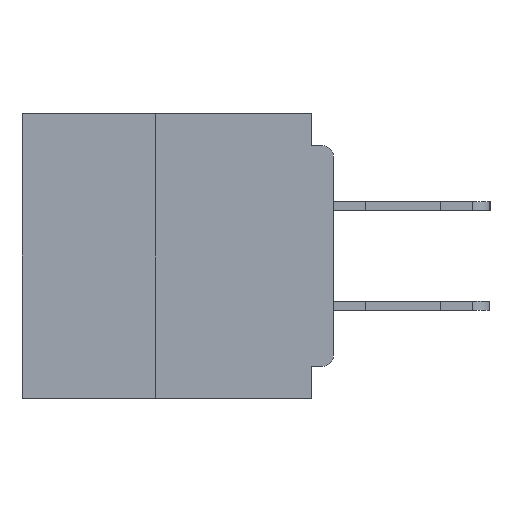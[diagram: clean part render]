
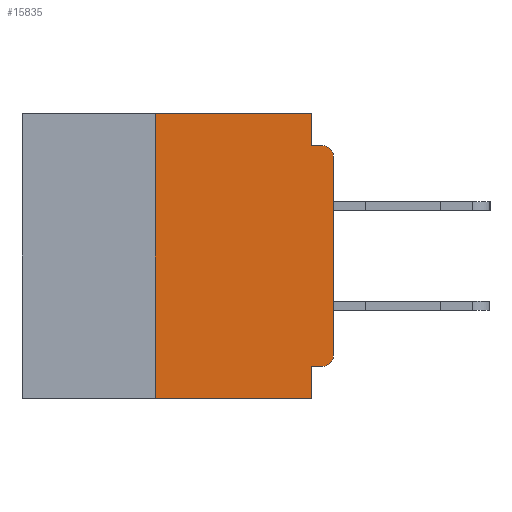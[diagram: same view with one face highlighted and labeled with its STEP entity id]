
A CAD part, left-side view. The second image highlights one B-rep face of the part: STEP entity #15835.
In plain terms, the highlighted planar face has unit normal (-1, 0, 0).
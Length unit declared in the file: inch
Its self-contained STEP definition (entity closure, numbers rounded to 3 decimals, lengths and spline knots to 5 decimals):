
#184 = VERTEX_POINT ( 'NONE', #32863 ) ;
#458 = CARTESIAN_POINT ( 'NONE',  ( 0., 0.015, -0.045 ) ) ;
#2667 = CARTESIAN_POINT ( 'NONE',  ( 0., 0.031, 0. ) ) ;
#2810 = FACE_OUTER_BOUND ( 'NONE', #41546, .T. ) ;
#3434 = CIRCLE ( 'NONE', #31598, 0.015 ) ;
#3658 = VERTEX_POINT ( 'NONE', #49305 ) ;
#4244 = CARTESIAN_POINT ( 'NONE',  ( 0., 0.437, 0. ) ) ;
#4909 = CARTESIAN_POINT ( 'NONE',  ( 0., 0.25, -0.4 ) ) ;
#6077 = ORIENTED_EDGE ( 'NONE', *, *, #34252, .F. ) ;
#7349 = LINE ( 'NONE', #2667, #27005 ) ;
#7924 = ORIENTED_EDGE ( 'NONE', *, *, #21182, .T. ) ;
#8232 = PLANE ( 'NONE',  #28793 ) ;
#9226 = EDGE_CURVE ( 'NONE', #35657, #3658, #7349, .T. ) ;
#10929 = VERTEX_POINT ( 'NONE', #26954 ) ;
#10947 = DIRECTION ( 'NONE',  ( 0., 0., 1. ) ) ;
#11020 = CARTESIAN_POINT ( 'NONE',  ( 0., 0., -0.34 ) ) ;
#11292 = EDGE_CURVE ( 'NONE', #10929, #184, #44527, .T. ) ;
#11544 = LINE ( 'NONE', #22974, #29898 ) ;
#11643 = ORIENTED_EDGE ( 'NONE', *, *, #29785, .F. ) ;
#12203 = DIRECTION ( 'NONE',  ( 0., 0., -1. ) ) ;
#12277 = ORIENTED_EDGE ( 'NONE', *, *, #48271, .F. ) ;
#13813 = LINE ( 'NONE', #38050, #43877 ) ;
#14488 = VECTOR ( 'NONE', #44711, 39.37008 ) ;
#15175 = DIRECTION ( 'NONE',  ( 0., -1., 0. ) ) ;
#15835 = ADVANCED_FACE ( 'NONE', ( #2810 ), #8232, .F. ) ;
#17308 = VECTOR ( 'NONE', #38250, 39.37008 ) ;
#17671 = CARTESIAN_POINT ( 'NONE',  ( 0., 0., -0.045 ) ) ;
#18034 = CARTESIAN_POINT ( 'NONE',  ( 0., 0.015, -0.06 ) ) ;
#19011 = VECTOR ( 'NONE', #10947, 39.37008 ) ;
#19071 = ORIENTED_EDGE ( 'NONE', *, *, #39873, .F. ) ;
#21097 = CARTESIAN_POINT ( 'NONE',  ( 0., 0.015, -0.34 ) ) ;
#21182 = EDGE_CURVE ( 'NONE', #34264, #40122, #50197, .T. ) ;
#21324 = CARTESIAN_POINT ( 'NONE',  ( 0., 0., -0.355 ) ) ;
#21983 = DIRECTION ( 'NONE',  ( 0., 0., -1. ) ) ;
#22974 = CARTESIAN_POINT ( 'NONE',  ( 0., 0.437, -0.4 ) ) ;
#23741 = LINE ( 'NONE', #4909, #42085 ) ;
#23980 = ORIENTED_EDGE ( 'NONE', *, *, #47363, .T. ) ;
#24059 = AXIS2_PLACEMENT_3D ( 'NONE', #18034, #45352, #21983 ) ;
#24980 = DIRECTION ( 'NONE',  ( 0., 0., -1. ) ) ;
#26954 = CARTESIAN_POINT ( 'NONE',  ( 0., 0.015, -0.355 ) ) ;
#27005 = VECTOR ( 'NONE', #34107, 39.37008 ) ;
#27513 = CIRCLE ( 'NONE', #24059, 0.015 ) ;
#28793 = AXIS2_PLACEMENT_3D ( 'NONE', #4244, #35649, #12203 ) ;
#29660 = VECTOR ( 'NONE', #45003, 39.37008 ) ;
#29785 = EDGE_CURVE ( 'NONE', #3658, #34527, #40076, .T. ) ;
#29898 = VECTOR ( 'NONE', #15175, 39.37008 ) ;
#30170 = CARTESIAN_POINT ( 'NONE',  ( 0., 0.25, 0. ) ) ;
#30468 = CARTESIAN_POINT ( 'NONE',  ( 0., 0., 0. ) ) ;
#31248 = ORIENTED_EDGE ( 'NONE', *, *, #46594, .T. ) ;
#31598 = AXIS2_PLACEMENT_3D ( 'NONE', #21097, #48409, #24980 ) ;
#32863 = CARTESIAN_POINT ( 'NONE',  ( 0., 0.031, -0.355 ) ) ;
#33064 = CARTESIAN_POINT ( 'NONE',  ( 0., 0.031, -0.4 ) ) ;
#34107 = DIRECTION ( 'NONE',  ( 0., 0., -1. ) ) ;
#34252 = EDGE_CURVE ( 'NONE', #48262, #35657, #48514, .T. ) ;
#34264 = VERTEX_POINT ( 'NONE', #11020 ) ;
#34327 = CARTESIAN_POINT ( 'NONE',  ( 0., 0.437, 0. ) ) ;
#34527 = VERTEX_POINT ( 'NONE', #458 ) ;
#34931 = ORIENTED_EDGE ( 'NONE', *, *, #9226, .F. ) ;
#35649 = DIRECTION ( 'NONE',  ( 1., 0., 0. ) ) ;
#35657 = VERTEX_POINT ( 'NONE', #45687 ) ;
#36324 = EDGE_CURVE ( 'NONE', #39149, #37345, #11544, .T. ) ;
#37345 = VERTEX_POINT ( 'NONE', #33064 ) ;
#37460 = CARTESIAN_POINT ( 'NONE',  ( 0., 0., -0.06 ) ) ;
#38050 = CARTESIAN_POINT ( 'NONE',  ( 0., 0.031, -0.4 ) ) ;
#38250 = DIRECTION ( 'NONE',  ( 0., -1., 0. ) ) ;
#39149 = VERTEX_POINT ( 'NONE', #47664 ) ;
#39873 = EDGE_CURVE ( 'NONE', #39149, #48262, #23741, .T. ) ;
#40076 = LINE ( 'NONE', #17671, #29660 ) ;
#40122 = VERTEX_POINT ( 'NONE', #37460 ) ;
#40228 = DIRECTION ( 'NONE',  ( 0., 0., 1. ) ) ;
#41546 = EDGE_LOOP ( 'NONE', ( #7924, #31248, #11643, #34931, #6077, #19071, #50257, #12277, #43552, #23980 ) ) ;
#42032 = DIRECTION ( 'NONE',  ( 0., 0., -1. ) ) ;
#42085 = VECTOR ( 'NONE', #40228, 39.37008 ) ;
#43552 = ORIENTED_EDGE ( 'NONE', *, *, #11292, .F. ) ;
#43877 = VECTOR ( 'NONE', #42032, 39.37008 ) ;
#44527 = LINE ( 'NONE', #21324, #14488 ) ;
#44711 = DIRECTION ( 'NONE',  ( 0., 1., 0. ) ) ;
#45003 = DIRECTION ( 'NONE',  ( 0., -1., 0. ) ) ;
#45352 = DIRECTION ( 'NONE',  ( -1., 0., 0. ) ) ;
#45687 = CARTESIAN_POINT ( 'NONE',  ( 0., 0.031, 0. ) ) ;
#46594 = EDGE_CURVE ( 'NONE', #40122, #34527, #27513, .T. ) ;
#47363 = EDGE_CURVE ( 'NONE', #10929, #34264, #3434, .T. ) ;
#47664 = CARTESIAN_POINT ( 'NONE',  ( 0., 0.25, -0.4 ) ) ;
#48262 = VERTEX_POINT ( 'NONE', #30170 ) ;
#48271 = EDGE_CURVE ( 'NONE', #184, #37345, #13813, .T. ) ;
#48409 = DIRECTION ( 'NONE',  ( -1., 0., 0. ) ) ;
#48514 = LINE ( 'NONE', #34327, #17308 ) ;
#49305 = CARTESIAN_POINT ( 'NONE',  ( 0., 0.031, -0.045 ) ) ;
#50197 = LINE ( 'NONE', #30468, #19011 ) ;
#50257 = ORIENTED_EDGE ( 'NONE', *, *, #36324, .T. ) ;
